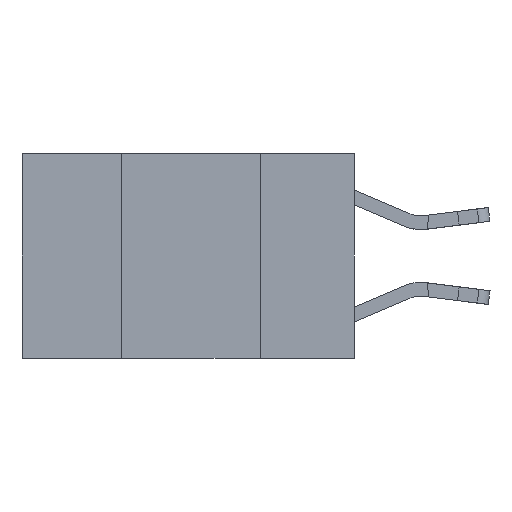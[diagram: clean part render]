
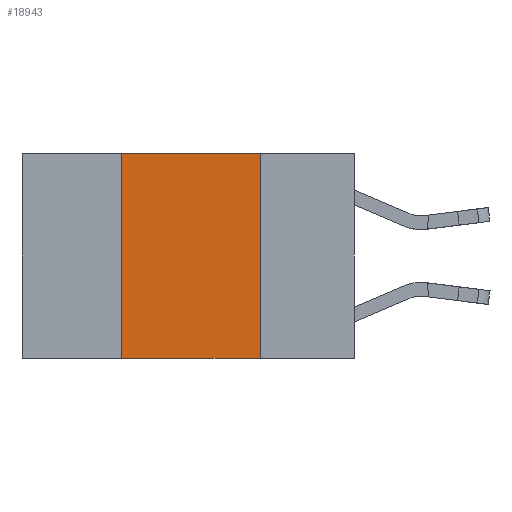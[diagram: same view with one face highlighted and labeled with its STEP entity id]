
A CAD part, left-side view. The second image highlights one B-rep face of the part: STEP entity #18943.
In plain terms, the highlighted planar face has unit normal (-1, 0, 0).
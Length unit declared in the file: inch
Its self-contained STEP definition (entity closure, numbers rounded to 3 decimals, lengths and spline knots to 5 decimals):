
#26 = VECTOR ( 'NONE', #13907, 39.37008 ) ;
#190 = FACE_OUTER_BOUND ( 'NONE', #19046, .T. ) ;
#516 = EDGE_CURVE ( 'NONE', #11146, #7914, #16188, .T. ) ;
#1387 = VERTEX_POINT ( 'NONE', #16082 ) ;
#1968 = VECTOR ( 'NONE', #9097, 39.37008 ) ;
#3214 = LINE ( 'NONE', #4846, #7156 ) ;
#3681 = CARTESIAN_POINT ( 'NONE',  ( 0., 0.42, -0.37 ) ) ;
#3946 = LINE ( 'NONE', #10525, #26 ) ;
#4831 = PLANE ( 'NONE',  #11869 ) ;
#4846 = CARTESIAN_POINT ( 'NONE',  ( 0., 0.42, 0. ) ) ;
#6354 = VERTEX_POINT ( 'NONE', #3681 ) ;
#6415 = EDGE_CURVE ( 'NONE', #1387, #11146, #3946, .T. ) ;
#6523 = DIRECTION ( 'NONE',  ( 0., 0., 1. ) ) ;
#7156 = VECTOR ( 'NONE', #6523, 39.37008 ) ;
#7416 = CARTESIAN_POINT ( 'NONE',  ( 0., 0.6, -0.37 ) ) ;
#7914 = VERTEX_POINT ( 'NONE', #17487 ) ;
#9097 = DIRECTION ( 'NONE',  ( 0., -1., 0. ) ) ;
#9893 = DIRECTION ( 'NONE',  ( 0., 0., -1. ) ) ;
#10525 = CARTESIAN_POINT ( 'NONE',  ( 0., 0.6, 0. ) ) ;
#11146 = VERTEX_POINT ( 'NONE', #19740 ) ;
#11516 = CARTESIAN_POINT ( 'NONE',  ( 0., 0.6, 0. ) ) ;
#11528 = ORIENTED_EDGE ( 'NONE', *, *, #516, .F. ) ;
#11869 = AXIS2_PLACEMENT_3D ( 'NONE', #11516, #19913, #9893 ) ;
#12083 = ORIENTED_EDGE ( 'NONE', *, *, #6415, .F. ) ;
#13362 = ORIENTED_EDGE ( 'NONE', *, *, #21134, .F. ) ;
#13907 = DIRECTION ( 'NONE',  ( 0., -1., 0. ) ) ;
#15345 = LINE ( 'NONE', #7416, #1968 ) ;
#15907 = ORIENTED_EDGE ( 'NONE', *, *, #20024, .T. ) ;
#16082 = CARTESIAN_POINT ( 'NONE',  ( 0., 0.42, 0. ) ) ;
#16188 = LINE ( 'NONE', #17109, #16218 ) ;
#16218 = VECTOR ( 'NONE', #16979, 39.37008 ) ;
#16979 = DIRECTION ( 'NONE',  ( 0., 0., -1. ) ) ;
#17109 = CARTESIAN_POINT ( 'NONE',  ( 0., 0.17, 0. ) ) ;
#17487 = CARTESIAN_POINT ( 'NONE',  ( 0., 0.17, -0.37 ) ) ;
#18943 = ADVANCED_FACE ( 'NONE', ( #190 ), #4831, .F. ) ;
#19046 = EDGE_LOOP ( 'NONE', ( #11528, #12083, #13362, #15907 ) ) ;
#19740 = CARTESIAN_POINT ( 'NONE',  ( 0., 0.17, 0. ) ) ;
#19913 = DIRECTION ( 'NONE',  ( 1., 0., 0. ) ) ;
#20024 = EDGE_CURVE ( 'NONE', #6354, #7914, #15345, .T. ) ;
#21134 = EDGE_CURVE ( 'NONE', #6354, #1387, #3214, .T. ) ;
